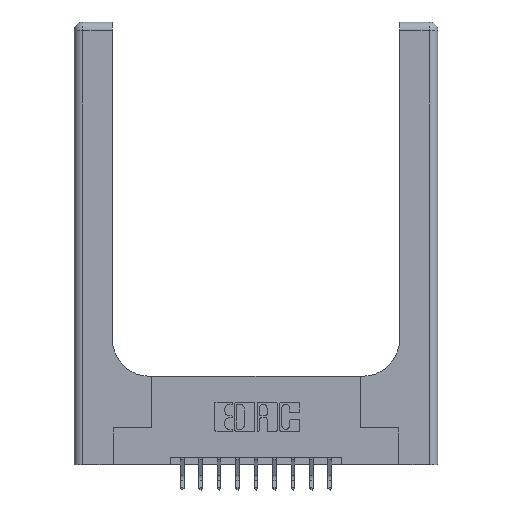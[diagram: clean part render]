
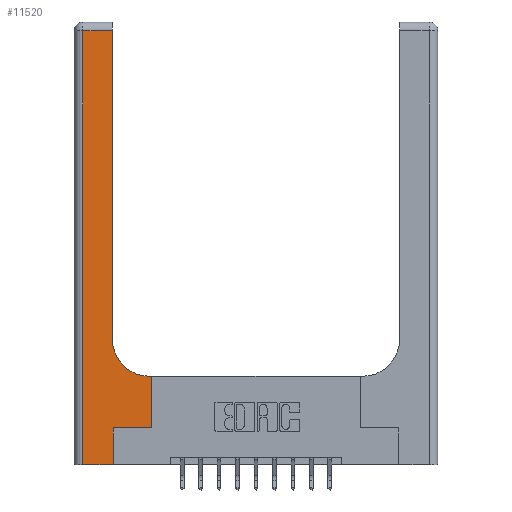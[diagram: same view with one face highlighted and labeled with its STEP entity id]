
A CAD part, top view. The second image highlights one B-rep face of the part: STEP entity #11520.
In plain terms, the highlighted planar face has unit normal (0, 0, 1).
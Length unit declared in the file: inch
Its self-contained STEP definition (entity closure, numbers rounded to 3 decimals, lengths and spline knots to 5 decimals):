
#279 = CARTESIAN_POINT ( 'NONE',  ( 0.528, 0.25, 0.37 ) ) ;
#341 = AXIS2_PLACEMENT_3D ( 'NONE', #4388, #10694, #15684 ) ;
#373 = VECTOR ( 'NONE', #8517, 39.37008 ) ;
#990 = LINE ( 'NONE', #9741, #373 ) ;
#1094 = ORIENTED_EDGE ( 'NONE', *, *, #9423, .T. ) ;
#1418 = DIRECTION ( 'NONE',  ( -1., 0., 0. ) ) ;
#1508 = VERTEX_POINT ( 'NONE', #8340 ) ;
#2510 = EDGE_CURVE ( 'NONE', #4921, #6097, #11869, .T. ) ;
#2629 = VECTOR ( 'NONE', #1418, 39.37008 ) ;
#2830 = CARTESIAN_POINT ( 'NONE',  ( 0., 0., 0.37 ) ) ;
#2994 = VECTOR ( 'NONE', #12806, 39.37008 ) ;
#4057 = CARTESIAN_POINT ( 'NONE',  ( 0.51, 0.6, 0.37 ) ) ;
#4143 = DIRECTION ( 'NONE',  ( 0., 0., -1. ) ) ;
#4216 = FACE_OUTER_BOUND ( 'NONE', #10591, .T. ) ;
#4246 = EDGE_CURVE ( 'NONE', #5055, #14543, #12361, .T. ) ;
#4388 = CARTESIAN_POINT ( 'NONE',  ( 0.51, 0.85, 0.37 ) ) ;
#4432 = CARTESIAN_POINT ( 'NONE',  ( 0.265, 0., 0.37 ) ) ;
#4790 = VECTOR ( 'NONE', #10741, 39.37008 ) ;
#4921 = VERTEX_POINT ( 'NONE', #13540 ) ;
#4979 = DIRECTION ( 'NONE',  ( -1., 0., 0. ) ) ;
#5055 = VERTEX_POINT ( 'NONE', #5181 ) ;
#5071 = CARTESIAN_POINT ( 'NONE',  ( 0.26, 0.6, 0.37 ) ) ;
#5181 = CARTESIAN_POINT ( 'NONE',  ( 0.528, 0.6, 0.37 ) ) ;
#5378 = DIRECTION ( 'NONE',  ( -1., 0., 0. ) ) ;
#5566 = CIRCLE ( 'NONE', #341, 0.25 ) ;
#5675 = CARTESIAN_POINT ( 'NONE',  ( 0.06, 0., 0.37 ) ) ;
#5907 = ORIENTED_EDGE ( 'NONE', *, *, #8550, .T. ) ;
#6013 = LINE ( 'NONE', #12145, #11620 ) ;
#6097 = VERTEX_POINT ( 'NONE', #5675 ) ;
#6264 = VECTOR ( 'NONE', #4979, 39.37008 ) ;
#6584 = VERTEX_POINT ( 'NONE', #11535 ) ;
#7758 = EDGE_CURVE ( 'NONE', #14543, #1508, #5566, .T. ) ;
#8340 = CARTESIAN_POINT ( 'NONE',  ( 0.26, 0.85, 0.37 ) ) ;
#8517 = DIRECTION ( 'NONE',  ( 1., 0., 0. ) ) ;
#8550 = EDGE_CURVE ( 'NONE', #10881, #9778, #10979, .T. ) ;
#8997 = CARTESIAN_POINT ( 'NONE',  ( 0.265, 0., 0.37 ) ) ;
#9137 = EDGE_CURVE ( 'NONE', #9778, #6584, #990, .T. ) ;
#9166 = ORIENTED_EDGE ( 'NONE', *, *, #13445, .T. ) ;
#9185 = VERTEX_POINT ( 'NONE', #15436 ) ;
#9423 = EDGE_CURVE ( 'NONE', #6097, #10881, #12972, .T. ) ;
#9717 = EDGE_CURVE ( 'NONE', #9185, #4921, #13854, .T. ) ;
#9741 = CARTESIAN_POINT ( 'NONE',  ( 0.265, 0.25, 0.37 ) ) ;
#9775 = DIRECTION ( 'NONE',  ( 0., 1., 0. ) ) ;
#9778 = VERTEX_POINT ( 'NONE', #14099 ) ;
#10510 = ORIENTED_EDGE ( 'NONE', *, *, #9717, .T. ) ;
#10543 = AXIS2_PLACEMENT_3D ( 'NONE', #11591, #4143, #5378 ) ;
#10591 = EDGE_LOOP ( 'NONE', ( #9166, #10510, #15790, #1094, #5907, #16150, #15090, #15819, #12674 ) ) ;
#10594 = VECTOR ( 'NONE', #13709, 39.37008 ) ;
#10694 = DIRECTION ( 'NONE',  ( 0., 0., -1. ) ) ;
#10741 = DIRECTION ( 'NONE',  ( 0., 1., 0. ) ) ;
#10881 = VERTEX_POINT ( 'NONE', #8997 ) ;
#10979 = LINE ( 'NONE', #4432, #4790 ) ;
#11520 = ADVANCED_FACE ( 'NONE', ( #4216 ), #12986, .F. ) ;
#11535 = CARTESIAN_POINT ( 'NONE',  ( 0.528, 0.25, 0.37 ) ) ;
#11591 = CARTESIAN_POINT ( 'NONE',  ( 0., 3., 0.37 ) ) ;
#11620 = VECTOR ( 'NONE', #9775, 39.37008 ) ;
#11869 = LINE ( 'NONE', #12937, #12292 ) ;
#12145 = CARTESIAN_POINT ( 'NONE',  ( 0.26, 3., 0.37 ) ) ;
#12292 = VECTOR ( 'NONE', #13009, 39.37008 ) ;
#12361 = LINE ( 'NONE', #5071, #6264 ) ;
#12631 = CARTESIAN_POINT ( 'NONE',  ( 0., 2.94, 0.37 ) ) ;
#12674 = ORIENTED_EDGE ( 'NONE', *, *, #7758, .T. ) ;
#12723 = LINE ( 'NONE', #279, #10594 ) ;
#12806 = DIRECTION ( 'NONE',  ( 1., 0., 0. ) ) ;
#12937 = CARTESIAN_POINT ( 'NONE',  ( 0.06, 3., 0.37 ) ) ;
#12972 = LINE ( 'NONE', #2830, #2994 ) ;
#12986 = PLANE ( 'NONE',  #10543 ) ;
#13009 = DIRECTION ( 'NONE',  ( 0., -1., 0. ) ) ;
#13445 = EDGE_CURVE ( 'NONE', #1508, #9185, #6013, .T. ) ;
#13540 = CARTESIAN_POINT ( 'NONE',  ( 0.06, 2.94, 0.37 ) ) ;
#13615 = EDGE_CURVE ( 'NONE', #6584, #5055, #12723, .T. ) ;
#13709 = DIRECTION ( 'NONE',  ( 0., 1., 0. ) ) ;
#13854 = LINE ( 'NONE', #12631, #2629 ) ;
#14099 = CARTESIAN_POINT ( 'NONE',  ( 0.265, 0.25, 0.37 ) ) ;
#14543 = VERTEX_POINT ( 'NONE', #4057 ) ;
#15090 = ORIENTED_EDGE ( 'NONE', *, *, #13615, .T. ) ;
#15436 = CARTESIAN_POINT ( 'NONE',  ( 0.26, 2.94, 0.37 ) ) ;
#15684 = DIRECTION ( 'NONE',  ( 1., 0., 0. ) ) ;
#15790 = ORIENTED_EDGE ( 'NONE', *, *, #2510, .T. ) ;
#15819 = ORIENTED_EDGE ( 'NONE', *, *, #4246, .T. ) ;
#16150 = ORIENTED_EDGE ( 'NONE', *, *, #9137, .T. ) ;
